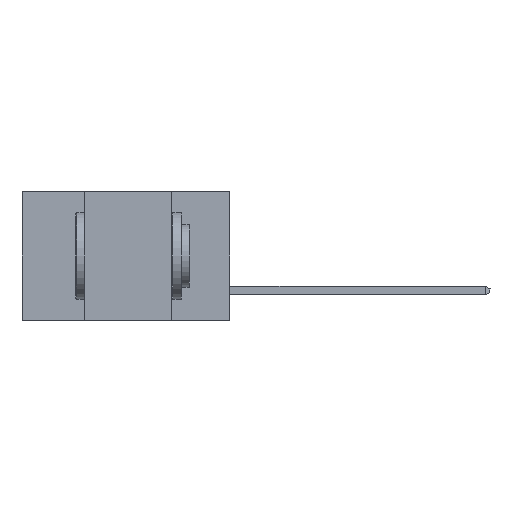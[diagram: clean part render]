
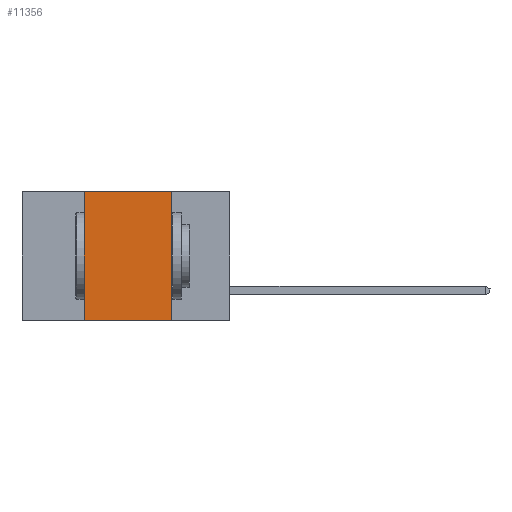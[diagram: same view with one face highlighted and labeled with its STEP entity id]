
A CAD part, left-side view. The second image highlights one B-rep face of the part: STEP entity #11356.
In plain terms, the highlighted planar face has unit normal (-1, 0, 0).
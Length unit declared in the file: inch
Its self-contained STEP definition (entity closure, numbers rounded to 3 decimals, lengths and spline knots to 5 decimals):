
#1060 = CARTESIAN_POINT ( 'NONE',  ( 0., 0.42, 0. ) ) ;
#1121 = ORIENTED_EDGE ( 'NONE', *, *, #1122, .F. ) ;
#1122 = EDGE_CURVE ( 'NONE', #10850, #17707, #1977, .T. ) ;
#1401 = CARTESIAN_POINT ( 'NONE',  ( 0., 0.6, 0. ) ) ;
#1515 = EDGE_CURVE ( 'NONE', #12870, #10850, #4209, .T. ) ;
#1871 = VERTEX_POINT ( 'NONE', #11399 ) ;
#1948 = VECTOR ( 'NONE', #6213, 39.37008 ) ;
#1977 = LINE ( 'NONE', #11920, #1948 ) ;
#2543 = PLANE ( 'NONE',  #17618 ) ;
#2986 = EDGE_LOOP ( 'NONE', ( #1121, #13712, #7052, #13358 ) ) ;
#3549 = CARTESIAN_POINT ( 'NONE',  ( 0., 0.17, 0. ) ) ;
#3608 = CARTESIAN_POINT ( 'NONE',  ( 0., 0.6, -0.37 ) ) ;
#3907 = CARTESIAN_POINT ( 'NONE',  ( 0., 0.6, 0. ) ) ;
#4209 = LINE ( 'NONE', #1401, #13370 ) ;
#4412 = CARTESIAN_POINT ( 'NONE',  ( 0., 0.17, -0.37 ) ) ;
#5150 = DIRECTION ( 'NONE',  ( 0., 0., -1. ) ) ;
#5676 = VECTOR ( 'NONE', #12366, 39.37008 ) ;
#5812 = CARTESIAN_POINT ( 'NONE',  ( 0., 0.42, -0.37 ) ) ;
#6213 = DIRECTION ( 'NONE',  ( 0., 0., -1. ) ) ;
#6594 = DIRECTION ( 'NONE',  ( 1., 0., 0. ) ) ;
#7052 = ORIENTED_EDGE ( 'NONE', *, *, #16923, .F. ) ;
#8344 = DIRECTION ( 'NONE',  ( 0., -1., 0. ) ) ;
#9864 = FACE_OUTER_BOUND ( 'NONE', #2986, .T. ) ;
#10342 = LINE ( 'NONE', #5812, #10654 ) ;
#10654 = VECTOR ( 'NONE', #13345, 39.37008 ) ;
#10850 = VERTEX_POINT ( 'NONE', #3549 ) ;
#11356 = ADVANCED_FACE ( 'NONE', ( #9864 ), #2543, .F. ) ;
#11399 = CARTESIAN_POINT ( 'NONE',  ( 0., 0.42, -0.37 ) ) ;
#11920 = CARTESIAN_POINT ( 'NONE',  ( 0., 0.17, -0.37 ) ) ;
#12366 = DIRECTION ( 'NONE',  ( 0., -1., 0. ) ) ;
#12870 = VERTEX_POINT ( 'NONE', #1060 ) ;
#13345 = DIRECTION ( 'NONE',  ( 0., 0., 1. ) ) ;
#13358 = ORIENTED_EDGE ( 'NONE', *, *, #13506, .T. ) ;
#13370 = VECTOR ( 'NONE', #8344, 39.37008 ) ;
#13506 = EDGE_CURVE ( 'NONE', #1871, #17707, #15374, .T. ) ;
#13712 = ORIENTED_EDGE ( 'NONE', *, *, #1515, .F. ) ;
#15374 = LINE ( 'NONE', #3608, #5676 ) ;
#16923 = EDGE_CURVE ( 'NONE', #1871, #12870, #10342, .T. ) ;
#17618 = AXIS2_PLACEMENT_3D ( 'NONE', #3907, #6594, #5150 ) ;
#17707 = VERTEX_POINT ( 'NONE', #4412 ) ;
